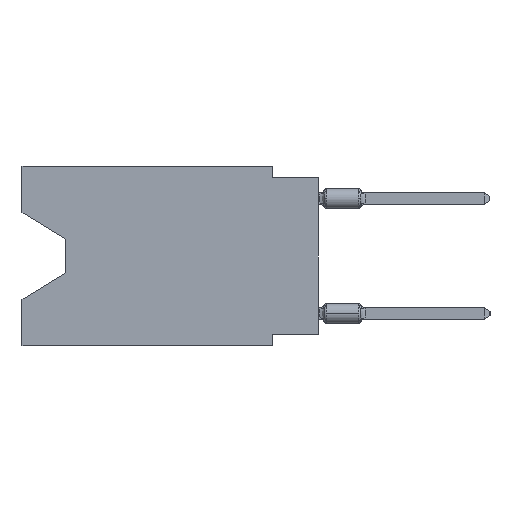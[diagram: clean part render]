
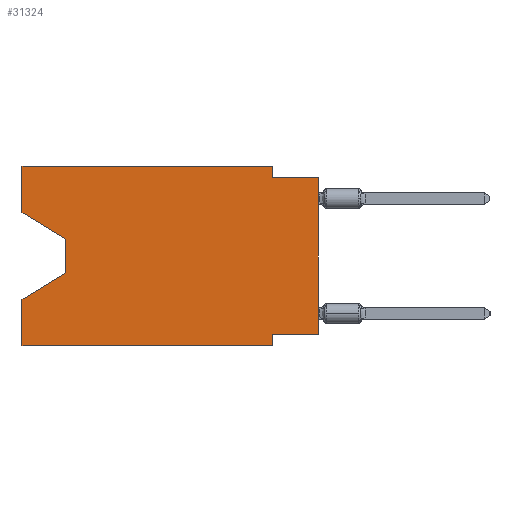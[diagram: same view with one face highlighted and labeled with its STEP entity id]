
A CAD part, left-side view. The second image highlights one B-rep face of the part: STEP entity #31324.
In plain terms, the highlighted planar face has unit normal (-1, 0, 0).
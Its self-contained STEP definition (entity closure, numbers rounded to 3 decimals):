
#431 = CARTESIAN_POINT ( 'NONE',  ( 0., 13.97, -4.013 ) ) ;
#528 = CARTESIAN_POINT ( 'NONE',  ( 0., 0., -0.635 ) ) ;
#551 = CARTESIAN_POINT ( 'NONE',  ( 0., 16.383, -2.546 ) ) ;
#1642 = CARTESIAN_POINT ( 'NONE',  ( 0., 2.54, -9.906 ) ) ;
#1739 = ORIENTED_EDGE ( 'NONE', *, *, #45472, .F. ) ;
#2144 = CARTESIAN_POINT ( 'NONE',  ( 0., 0., -9.271 ) ) ;
#2615 = DIRECTION ( 'NONE',  ( 0., -1., 0. ) ) ;
#3141 = VECTOR ( 'NONE', #56725, 1000. ) ;
#3891 = CARTESIAN_POINT ( 'NONE',  ( 0., 16.383, -9.906 ) ) ;
#4426 = VERTEX_POINT ( 'NONE', #6089 ) ;
#4969 = CARTESIAN_POINT ( 'NONE',  ( 0., 2.54, 0. ) ) ;
#5049 = CARTESIAN_POINT ( 'NONE',  ( 0., 16.383, 0. ) ) ;
#5661 = CARTESIAN_POINT ( 'NONE',  ( 0., 2.54, -9.271 ) ) ;
#5782 = CARTESIAN_POINT ( 'NONE',  ( 0., 16.383, 0. ) ) ;
#6007 = EDGE_CURVE ( 'NONE', #28139, #11044, #33364, .T. ) ;
#6089 = CARTESIAN_POINT ( 'NONE',  ( 0., 13.97, -5.893 ) ) ;
#7509 = DIRECTION ( 'NONE',  ( 0., 0., 1. ) ) ;
#7717 = VERTEX_POINT ( 'NONE', #24842 ) ;
#8183 = EDGE_LOOP ( 'NONE', ( #45551, #56755, #25902, #30061, #43964, #54893, #33630, #52009, #32413, #22220, #1739, #30094 ) ) ;
#8755 = DIRECTION ( 'NONE',  ( 0., 0., -1. ) ) ;
#9594 = CARTESIAN_POINT ( 'NONE',  ( 0., 0., -9.271 ) ) ;
#11044 = VERTEX_POINT ( 'NONE', #37321 ) ;
#11152 = VERTEX_POINT ( 'NONE', #24711 ) ;
#11685 = LINE ( 'NONE', #43292, #44487 ) ;
#12301 = VECTOR ( 'NONE', #7509, 1000. ) ;
#12364 = EDGE_CURVE ( 'NONE', #15790, #59462, #35577, .T. ) ;
#13113 = EDGE_CURVE ( 'NONE', #59462, #28229, #53153, .T. ) ;
#13252 = VECTOR ( 'NONE', #8755, 1000. ) ;
#13260 = VERTEX_POINT ( 'NONE', #31348 ) ;
#15495 = LINE ( 'NONE', #40924, #59027 ) ;
#15790 = VERTEX_POINT ( 'NONE', #9594 ) ;
#15844 = VECTOR ( 'NONE', #48056, 1000. ) ;
#16511 = CARTESIAN_POINT ( 'NONE',  ( 0., 16.383, -7.36 ) ) ;
#17006 = LINE ( 'NONE', #41246, #12301 ) ;
#17443 = FACE_OUTER_BOUND ( 'NONE', #8183, .T. ) ;
#18074 = VECTOR ( 'NONE', #27427, 1000. ) ;
#18854 = CARTESIAN_POINT ( 'NONE',  ( 0., 2.54, 0. ) ) ;
#21969 = EDGE_CURVE ( 'NONE', #7717, #28229, #46828, .T. ) ;
#22026 = VECTOR ( 'NONE', #34769, 1000. ) ;
#22220 = ORIENTED_EDGE ( 'NONE', *, *, #40828, .F. ) ;
#23821 = LINE ( 'NONE', #528, #15844 ) ;
#23915 = VECTOR ( 'NONE', #31558, 1000. ) ;
#24110 = EDGE_CURVE ( 'NONE', #11044, #4426, #42444, .T. ) ;
#24711 = CARTESIAN_POINT ( 'NONE',  ( 0., 0., -0.635 ) ) ;
#24842 = CARTESIAN_POINT ( 'NONE',  ( 0., 16.383, -9.906 ) ) ;
#25124 = EDGE_CURVE ( 'NONE', #28139, #55451, #17006, .T. ) ;
#25902 = ORIENTED_EDGE ( 'NONE', *, *, #27315, .T. ) ;
#26353 = PLANE ( 'NONE',  #40597 ) ;
#26355 = VERTEX_POINT ( 'NONE', #16511 ) ;
#26591 = EDGE_CURVE ( 'NONE', #13260, #11152, #23821, .T. ) ;
#27315 = EDGE_CURVE ( 'NONE', #4426, #26355, #38039, .T. ) ;
#27427 = DIRECTION ( 'NONE',  ( 0., 0., -1. ) ) ;
#28139 = VERTEX_POINT ( 'NONE', #47314 ) ;
#28229 = VERTEX_POINT ( 'NONE', #29822 ) ;
#29822 = CARTESIAN_POINT ( 'NONE',  ( 0., 2.54, -9.906 ) ) ;
#30061 = ORIENTED_EDGE ( 'NONE', *, *, #36062, .F. ) ;
#30094 = ORIENTED_EDGE ( 'NONE', *, *, #25124, .F. ) ;
#30397 = DIRECTION ( 'NONE',  ( 0., 0., 1. ) ) ;
#31268 = CARTESIAN_POINT ( 'NONE',  ( 0., 16.383, 0. ) ) ;
#31324 = ADVANCED_FACE ( 'NONE', ( #17443 ), #26353, .F. ) ;
#31348 = CARTESIAN_POINT ( 'NONE',  ( 0., 2.54, -0.635 ) ) ;
#31558 = DIRECTION ( 'NONE',  ( 0., 1., 0. ) ) ;
#32413 = ORIENTED_EDGE ( 'NONE', *, *, #26591, .F. ) ;
#32811 = VERTEX_POINT ( 'NONE', #4969 ) ;
#33364 = LINE ( 'NONE', #551, #48292 ) ;
#33630 = ORIENTED_EDGE ( 'NONE', *, *, #12364, .F. ) ;
#34769 = DIRECTION ( 'NONE',  ( 0., 0., -1. ) ) ;
#35577 = LINE ( 'NONE', #2144, #23915 ) ;
#36062 = EDGE_CURVE ( 'NONE', #7717, #26355, #15495, .T. ) ;
#37301 = LINE ( 'NONE', #18854, #13252 ) ;
#37321 = CARTESIAN_POINT ( 'NONE',  ( 0., 13.97, -4.013 ) ) ;
#38039 = LINE ( 'NONE', #42627, #3141 ) ;
#38884 = DIRECTION ( 'NONE',  ( 0., -0.855, -0.519 ) ) ;
#40597 = AXIS2_PLACEMENT_3D ( 'NONE', #31268, #59781, #49968 ) ;
#40828 = EDGE_CURVE ( 'NONE', #32811, #13260, #37301, .T. ) ;
#40924 = CARTESIAN_POINT ( 'NONE',  ( 0., 16.383, 0. ) ) ;
#41246 = CARTESIAN_POINT ( 'NONE',  ( 0., 16.383, 0. ) ) ;
#42444 = LINE ( 'NONE', #431, #18074 ) ;
#42627 = CARTESIAN_POINT ( 'NONE',  ( 0., 13.97, -5.893 ) ) ;
#43292 = CARTESIAN_POINT ( 'NONE',  ( 0., 0., 0. ) ) ;
#43964 = ORIENTED_EDGE ( 'NONE', *, *, #21969, .T. ) ;
#44487 = VECTOR ( 'NONE', #30397, 1000. ) ;
#44654 = LINE ( 'NONE', #5782, #52806 ) ;
#45472 = EDGE_CURVE ( 'NONE', #55451, #32811, #44654, .T. ) ;
#45551 = ORIENTED_EDGE ( 'NONE', *, *, #6007, .T. ) ;
#46233 = EDGE_CURVE ( 'NONE', #15790, #11152, #11685, .T. ) ;
#46828 = LINE ( 'NONE', #3891, #59208 ) ;
#47314 = CARTESIAN_POINT ( 'NONE',  ( 0., 16.383, -2.546 ) ) ;
#48056 = DIRECTION ( 'NONE',  ( 0., -1., 0. ) ) ;
#48292 = VECTOR ( 'NONE', #38884, 1000. ) ;
#49818 = DIRECTION ( 'NONE',  ( 0., 0., 1. ) ) ;
#49968 = DIRECTION ( 'NONE',  ( 0., 0., -1. ) ) ;
#51428 = DIRECTION ( 'NONE',  ( 0., -1., 0. ) ) ;
#52009 = ORIENTED_EDGE ( 'NONE', *, *, #46233, .T. ) ;
#52806 = VECTOR ( 'NONE', #2615, 1000. ) ;
#53153 = LINE ( 'NONE', #1642, #22026 ) ;
#54893 = ORIENTED_EDGE ( 'NONE', *, *, #13113, .F. ) ;
#55451 = VERTEX_POINT ( 'NONE', #5049 ) ;
#56725 = DIRECTION ( 'NONE',  ( 0., 0.855, -0.519 ) ) ;
#56755 = ORIENTED_EDGE ( 'NONE', *, *, #24110, .T. ) ;
#59027 = VECTOR ( 'NONE', #49818, 1000. ) ;
#59208 = VECTOR ( 'NONE', #51428, 1000. ) ;
#59462 = VERTEX_POINT ( 'NONE', #5661 ) ;
#59781 = DIRECTION ( 'NONE',  ( 1., 0., 0. ) ) ;
